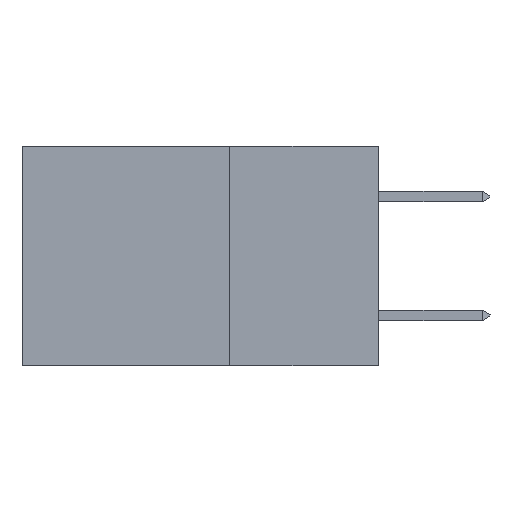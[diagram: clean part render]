
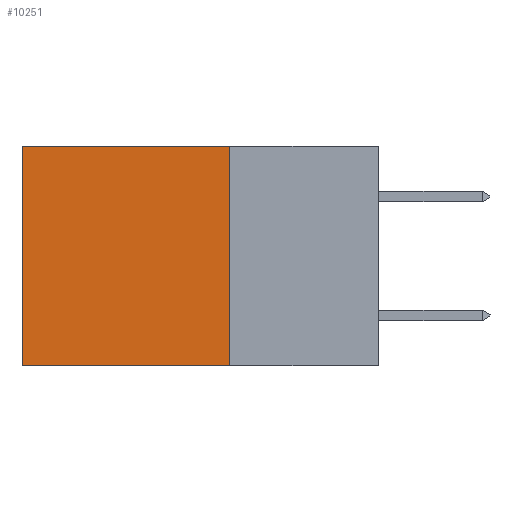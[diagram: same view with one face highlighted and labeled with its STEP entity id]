
A CAD part, left-side view. The second image highlights one B-rep face of the part: STEP entity #10251.
In plain terms, the highlighted planar face has unit normal (-1, 0, 0).
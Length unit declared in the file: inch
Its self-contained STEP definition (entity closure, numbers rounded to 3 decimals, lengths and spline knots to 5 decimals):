
#188 = DIRECTION ( 'NONE',  ( 0., 0., -1. ) ) ;
#2214 = LINE ( 'NONE', #15292, #8035 ) ;
#2422 = VERTEX_POINT ( 'NONE', #4358 ) ;
#2978 = DIRECTION ( 'NONE',  ( 0., 1., 0. ) ) ;
#4358 = CARTESIAN_POINT ( 'NONE',  ( 0.298, 0.6, -0.37 ) ) ;
#5116 = FACE_OUTER_BOUND ( 'NONE', #11640, .T. ) ;
#5756 = VECTOR ( 'NONE', #25792, 39.37008 ) ;
#6626 = CARTESIAN_POINT ( 'NONE',  ( 0.298, 0.25, -0.37 ) ) ;
#7625 = DIRECTION ( 'NONE',  ( 1., 0., 0. ) ) ;
#8035 = VECTOR ( 'NONE', #2978, 39.37008 ) ;
#9052 = CARTESIAN_POINT ( 'NONE',  ( 0.298, 0.6, 0. ) ) ;
#9247 = VERTEX_POINT ( 'NONE', #18183 ) ;
#9312 = LINE ( 'NONE', #6626, #21359 ) ;
#10169 = VERTEX_POINT ( 'NONE', #28868 ) ;
#10251 = ADVANCED_FACE ( 'NONE', ( #5116 ), #29168, .F. ) ;
#11117 = DIRECTION ( 'NONE',  ( 0., 0., -1. ) ) ;
#11640 = EDGE_LOOP ( 'NONE', ( #12221, #26366, #16733, #15443 ) ) ;
#11725 = VERTEX_POINT ( 'NONE', #30454 ) ;
#12221 = ORIENTED_EDGE ( 'NONE', *, *, #12413, .T. ) ;
#12413 = EDGE_CURVE ( 'NONE', #11725, #2422, #24161, .T. ) ;
#13935 = DIRECTION ( 'NONE',  ( 0., 1., 0. ) ) ;
#14270 = EDGE_CURVE ( 'NONE', #10169, #9247, #28586, .T. ) ;
#15067 = EDGE_CURVE ( 'NONE', #10169, #11725, #2214, .T. ) ;
#15087 = AXIS2_PLACEMENT_3D ( 'NONE', #26757, #7625, #188 ) ;
#15292 = CARTESIAN_POINT ( 'NONE',  ( 0.298, 0.25, 0. ) ) ;
#15443 = ORIENTED_EDGE ( 'NONE', *, *, #15067, .T. ) ;
#16733 = ORIENTED_EDGE ( 'NONE', *, *, #14270, .F. ) ;
#18080 = EDGE_CURVE ( 'NONE', #9247, #2422, #9312, .T. ) ;
#18183 = CARTESIAN_POINT ( 'NONE',  ( 0.298, 0.25, -0.37 ) ) ;
#21359 = VECTOR ( 'NONE', #13935, 39.37008 ) ;
#22995 = CARTESIAN_POINT ( 'NONE',  ( 0.298, 0.25, 0. ) ) ;
#24161 = LINE ( 'NONE', #9052, #5756 ) ;
#25792 = DIRECTION ( 'NONE',  ( 0., 0., -1. ) ) ;
#26366 = ORIENTED_EDGE ( 'NONE', *, *, #18080, .F. ) ;
#26757 = CARTESIAN_POINT ( 'NONE',  ( 0.298, 0.25, 0. ) ) ;
#27853 = VECTOR ( 'NONE', #11117, 39.37008 ) ;
#28586 = LINE ( 'NONE', #22995, #27853 ) ;
#28868 = CARTESIAN_POINT ( 'NONE',  ( 0.298, 0.25, 0. ) ) ;
#29168 = PLANE ( 'NONE',  #15087 ) ;
#30454 = CARTESIAN_POINT ( 'NONE',  ( 0.298, 0.6, 0. ) ) ;
